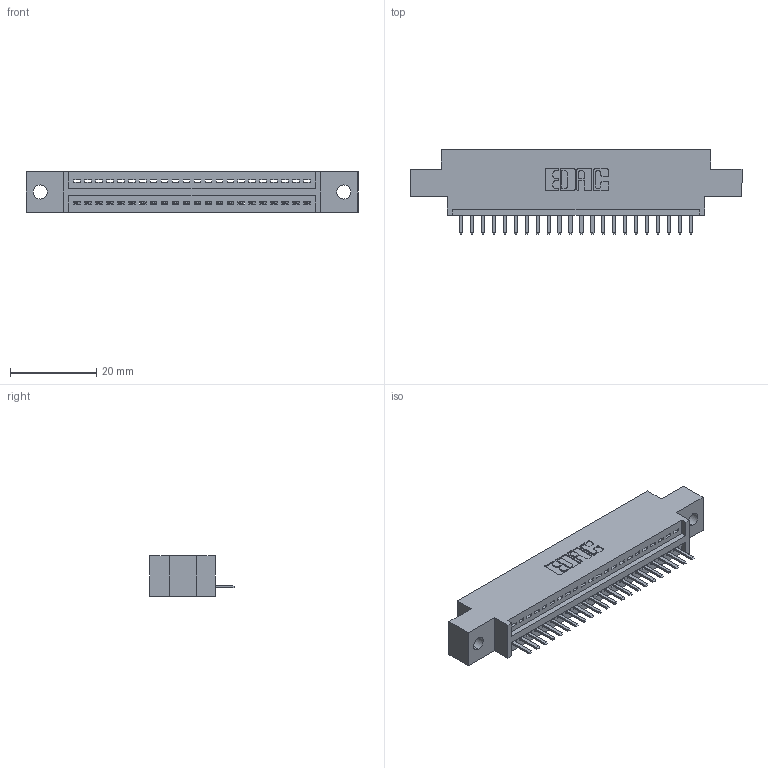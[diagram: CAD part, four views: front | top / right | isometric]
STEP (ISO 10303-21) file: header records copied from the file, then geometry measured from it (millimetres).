
FILE_DESCRIPTION (( 'STEP AP203' ), '1' );
FILE_NAME ('395-022-520-602.STEP', '2018-11-08T00:26:23', ( '' ), ( '' ), 'SwSTEP 2.0', 'SolidWorks 2016', '' );
FILE_SCHEMA (( 'CONFIG_CONTROL_DESIGN' ));
Length unit declared in the file: inch
Products named in the file (3): 345 Part_0.170 Offset - 0.128 Dia; 395-022-520-602; 345-292-001_345-293-120
Assembly tree (23 placements, depth 2):
  395-022-520-602
    345 Part_0.170 Offset - 0.128 Dia
    345-292-001_345-293-120  x22
Bounding box: 77.09 x 19.68 x 9.4 mm (x, y, z)
Volume: 6944.8 mm3; surface area: 8605.2 mm2
Topology: 23 solids, 23 shells, 1494 faces, 4401 edges, 2874 vertices
Faces by surface type: plane 1008, cylinder 486
Entity records: 19499 total; most frequent: CARTESIAN_POINT 3398, ORIENTED_EDGE 3342, DIRECTION 2983, EDGE_CURVE 1671, VECTOR 1447, LINE 1447, VERTEX_POINT 1110, AXIS2_PLACEMENT_3D 768
